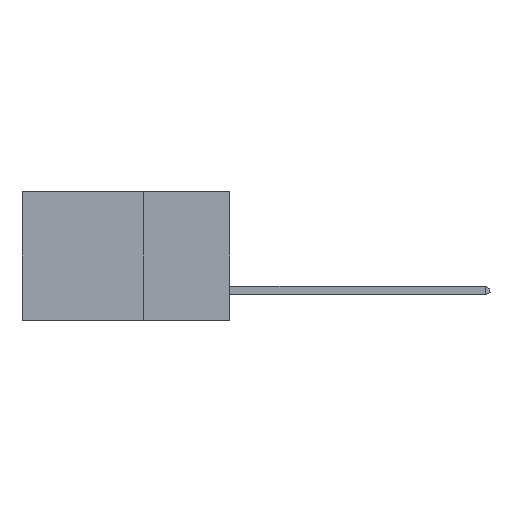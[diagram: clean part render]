
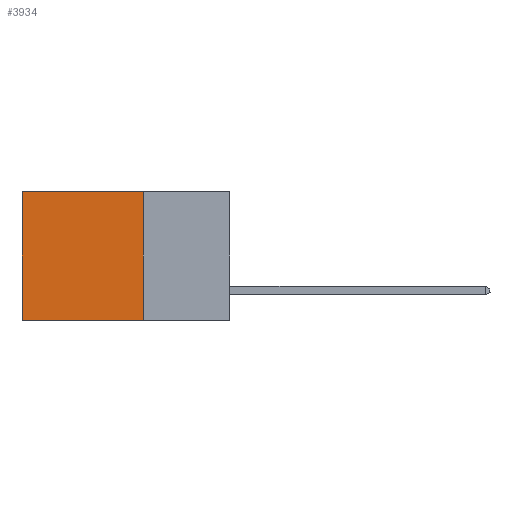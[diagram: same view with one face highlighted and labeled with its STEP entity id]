
A CAD part, left-side view. The second image highlights one B-rep face of the part: STEP entity #3934.
In plain terms, the highlighted planar face has unit normal (-1, 0, 0).
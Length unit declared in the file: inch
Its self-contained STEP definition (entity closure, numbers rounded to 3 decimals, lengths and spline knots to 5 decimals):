
#20 = FACE_OUTER_BOUND ( 'NONE', #6214, .T. ) ;
#146 = VECTOR ( 'NONE', #3563, 39.37008 ) ;
#347 = CARTESIAN_POINT ( 'NONE',  ( 0.298, 0.25, 0. ) ) ;
#405 = AXIS2_PLACEMENT_3D ( 'NONE', #2871, #12596, #2913 ) ;
#451 = CARTESIAN_POINT ( 'NONE',  ( 0.298, 0.25, 0. ) ) ;
#765 = CARTESIAN_POINT ( 'NONE',  ( 0.298, 0.25, -0.37 ) ) ;
#1028 = VECTOR ( 'NONE', #12637, 39.37008 ) ;
#2515 = ORIENTED_EDGE ( 'NONE', *, *, #5371, .T. ) ;
#2871 = CARTESIAN_POINT ( 'NONE',  ( 0.298, 0.25, 0. ) ) ;
#2913 = DIRECTION ( 'NONE',  ( 0., 0., -1. ) ) ;
#3563 = DIRECTION ( 'NONE',  ( 0., 0., -1. ) ) ;
#3934 = ADVANCED_FACE ( 'NONE', ( #20 ), #11618, .F. ) ;
#4043 = VERTEX_POINT ( 'NONE', #11176 ) ;
#4384 = CARTESIAN_POINT ( 'NONE',  ( 0.298, 0.25, -0.37 ) ) ;
#5074 = ORIENTED_EDGE ( 'NONE', *, *, #12096, .F. ) ;
#5371 = EDGE_CURVE ( 'NONE', #4043, #9715, #7606, .T. ) ;
#6214 = EDGE_LOOP ( 'NONE', ( #2515, #7619, #5074, #9613 ) ) ;
#6723 = VECTOR ( 'NONE', #12469, 39.37008 ) ;
#6959 = LINE ( 'NONE', #8805, #1028 ) ;
#7606 = LINE ( 'NONE', #8622, #146 ) ;
#7619 = ORIENTED_EDGE ( 'NONE', *, *, #10608, .F. ) ;
#8023 = VERTEX_POINT ( 'NONE', #4384 ) ;
#8085 = DIRECTION ( 'NONE',  ( 0., 1., 0. ) ) ;
#8622 = CARTESIAN_POINT ( 'NONE',  ( 0.298, 0.6, 0. ) ) ;
#8805 = CARTESIAN_POINT ( 'NONE',  ( 0.298, 0.25, 0. ) ) ;
#9200 = LINE ( 'NONE', #765, #6723 ) ;
#9613 = ORIENTED_EDGE ( 'NONE', *, *, #9959, .T. ) ;
#9715 = VERTEX_POINT ( 'NONE', #9752 ) ;
#9752 = CARTESIAN_POINT ( 'NONE',  ( 0.298, 0.6, -0.37 ) ) ;
#9959 = EDGE_CURVE ( 'NONE', #12361, #4043, #11038, .T. ) ;
#10097 = VECTOR ( 'NONE', #8085, 39.37008 ) ;
#10608 = EDGE_CURVE ( 'NONE', #8023, #9715, #9200, .T. ) ;
#11038 = LINE ( 'NONE', #451, #10097 ) ;
#11176 = CARTESIAN_POINT ( 'NONE',  ( 0.298, 0.6, 0. ) ) ;
#11618 = PLANE ( 'NONE',  #405 ) ;
#12096 = EDGE_CURVE ( 'NONE', #12361, #8023, #6959, .T. ) ;
#12361 = VERTEX_POINT ( 'NONE', #347 ) ;
#12469 = DIRECTION ( 'NONE',  ( 0., 1., 0. ) ) ;
#12596 = DIRECTION ( 'NONE',  ( 1., 0., 0. ) ) ;
#12637 = DIRECTION ( 'NONE',  ( 0., 0., -1. ) ) ;
